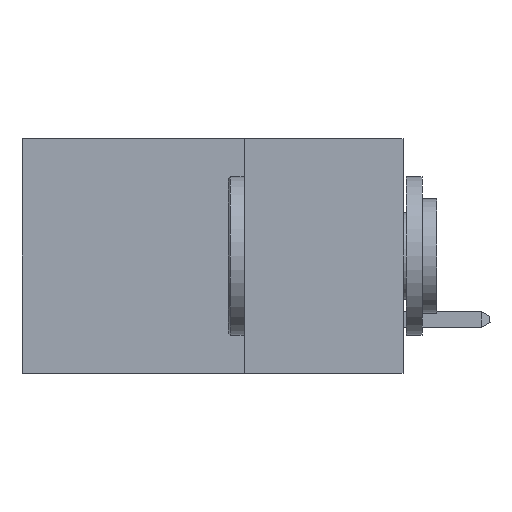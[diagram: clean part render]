
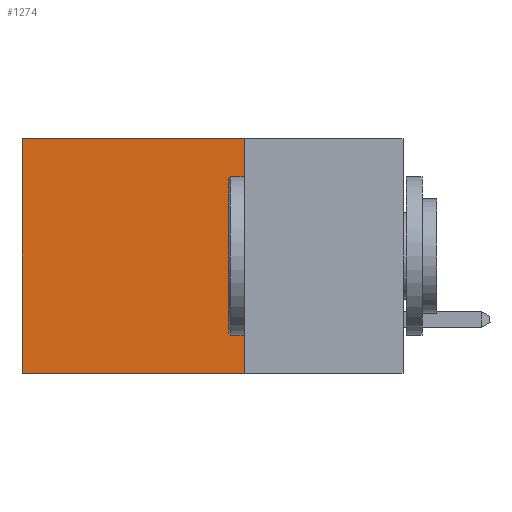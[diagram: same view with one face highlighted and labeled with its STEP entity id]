
A CAD part, left-side view. The second image highlights one B-rep face of the part: STEP entity #1274.
In plain terms, the highlighted planar face has unit normal (-1, 0, 0).
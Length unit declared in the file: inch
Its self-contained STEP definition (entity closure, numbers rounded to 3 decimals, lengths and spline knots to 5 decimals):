
#706 = VERTEX_POINT ( 'NONE', #15750 ) ;
#1274 = ADVANCED_FACE ( 'NONE', ( #10693 ), #6476, .F. ) ;
#2357 = EDGE_CURVE ( 'NONE', #20038, #3369, #19113, .T. ) ;
#3008 = EDGE_CURVE ( 'NONE', #3369, #12037, #3921, .T. ) ;
#3369 = VERTEX_POINT ( 'NONE', #16967 ) ;
#3921 = LINE ( 'NONE', #8879, #7920 ) ;
#4079 = VECTOR ( 'NONE', #4995, 39.37008 ) ;
#4300 = VECTOR ( 'NONE', #11864, 39.37008 ) ;
#4736 = DIRECTION ( 'NONE',  ( 1., 0., 0. ) ) ;
#4955 = LINE ( 'NONE', #15976, #18125 ) ;
#4995 = DIRECTION ( 'NONE',  ( 0., 0., -1. ) ) ;
#6476 = PLANE ( 'NONE',  #11468 ) ;
#6612 = CARTESIAN_POINT ( 'NONE',  ( 0.2875, 0.25, 0. ) ) ;
#7149 = DIRECTION ( 'NONE',  ( 0., 0., -1. ) ) ;
#7178 = CARTESIAN_POINT ( 'NONE',  ( 0.2875, 0.25, 0. ) ) ;
#7920 = VECTOR ( 'NONE', #7149, 39.37008 ) ;
#8692 = EDGE_LOOP ( 'NONE', ( #16130, #13644, #12597, #15515 ) ) ;
#8879 = CARTESIAN_POINT ( 'NONE',  ( 0.2875, 0.6, 0. ) ) ;
#10527 = EDGE_CURVE ( 'NONE', #20038, #706, #17274, .T. ) ;
#10693 = FACE_OUTER_BOUND ( 'NONE', #8692, .T. ) ;
#11468 = AXIS2_PLACEMENT_3D ( 'NONE', #6612, #4736, #14424 ) ;
#11864 = DIRECTION ( 'NONE',  ( 0., 1., 0. ) ) ;
#12037 = VERTEX_POINT ( 'NONE', #12771 ) ;
#12238 = CARTESIAN_POINT ( 'NONE',  ( 0.2875, 0.25, 0. ) ) ;
#12597 = ORIENTED_EDGE ( 'NONE', *, *, #10527, .F. ) ;
#12771 = CARTESIAN_POINT ( 'NONE',  ( 0.2875, 0.6, -0.37 ) ) ;
#12839 = DIRECTION ( 'NONE',  ( 0., 1., 0. ) ) ;
#13644 = ORIENTED_EDGE ( 'NONE', *, *, #16403, .F. ) ;
#14424 = DIRECTION ( 'NONE',  ( 0., 0., -1. ) ) ;
#15515 = ORIENTED_EDGE ( 'NONE', *, *, #2357, .T. ) ;
#15750 = CARTESIAN_POINT ( 'NONE',  ( 0.2875, 0.25, -0.37 ) ) ;
#15976 = CARTESIAN_POINT ( 'NONE',  ( 0.2875, 0.25, -0.37 ) ) ;
#16130 = ORIENTED_EDGE ( 'NONE', *, *, #3008, .T. ) ;
#16403 = EDGE_CURVE ( 'NONE', #706, #12037, #4955, .T. ) ;
#16967 = CARTESIAN_POINT ( 'NONE',  ( 0.2875, 0.6, 0. ) ) ;
#17274 = LINE ( 'NONE', #17697, #4079 ) ;
#17697 = CARTESIAN_POINT ( 'NONE',  ( 0.2875, 0.25, 0. ) ) ;
#18125 = VECTOR ( 'NONE', #12839, 39.37008 ) ;
#19113 = LINE ( 'NONE', #7178, #4300 ) ;
#20038 = VERTEX_POINT ( 'NONE', #12238 ) ;
